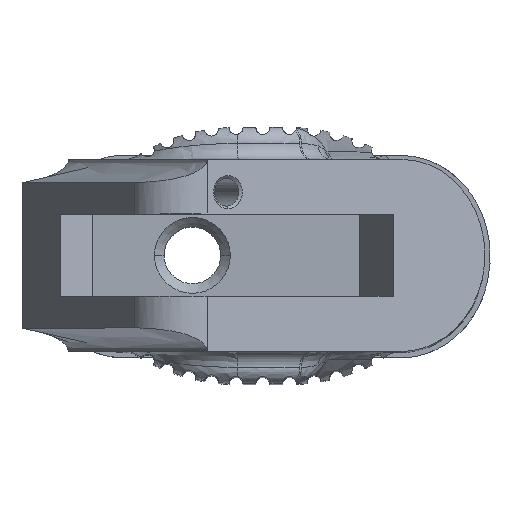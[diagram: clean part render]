
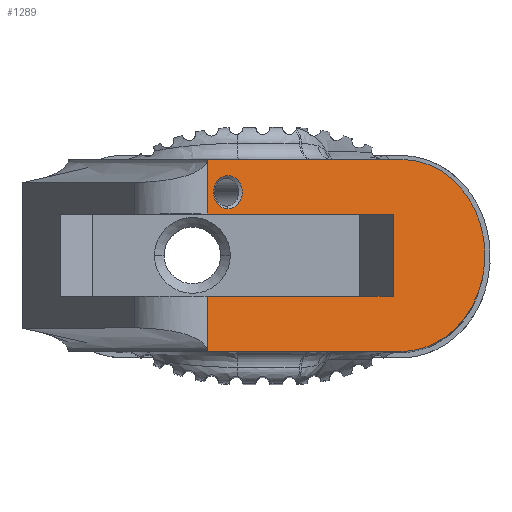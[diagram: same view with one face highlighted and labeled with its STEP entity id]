
A CAD part, top view. The second image highlights one B-rep face of the part: STEP entity #1289.
In plain terms, the highlighted planar face has unit normal (0.5, 0, 0.866).
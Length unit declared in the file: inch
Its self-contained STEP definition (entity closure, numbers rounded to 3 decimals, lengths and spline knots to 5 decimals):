
#49 = CARTESIAN_POINT ( 'NONE',  ( 0.64959, -1.00968, 2.3827 ) ) ;
#59 = CARTESIAN_POINT ( 'NONE',  ( 0.55214, -0.85579, 2.43896 ) ) ;
#67 = VERTEX_POINT ( 'NONE', #2289 ) ;
#109 = EDGE_CURVE ( 'NONE', #5710, #8721, #5941, .T. ) ;
#143 = CIRCLE ( 'NONE', #995, 0.07753 ) ;
#194 = LINE ( 'NONE', #4719, #1445 ) ;
#231 = VERTEX_POINT ( 'NONE', #6313 ) ;
#280 = CARTESIAN_POINT ( 'NONE',  ( 1.85118, -1.75318, 1.68896 ) ) ;
#450 = ORIENTED_EDGE ( 'NONE', *, *, #4851, .T. ) ;
#474 = CARTESIAN_POINT ( 'NONE',  ( 1.85118, -0.85518, 1.68896 ) ) ;
#483 = DIRECTION ( 'NONE',  ( 0., -1., 0. ) ) ;
#579 =( BOUNDED_CURVE ( )  B_SPLINE_CURVE ( 3, ( #3923, #6057, #5394, #5427 ),
 .UNSPECIFIED., .F., .F. ) 
 B_SPLINE_CURVE_WITH_KNOTS ( ( 4, 4 ),
 ( 0.00005, 0.01728 ),
 .UNSPECIFIED. ) 
 CURVE ( )  GEOMETRIC_REPRESENTATION_ITEM ( )  RATIONAL_B_SPLINE_CURVE ( ( 0.998, 0.813, 0.805, 0.974 ) ) 
 REPRESENTATION_ITEM ( '' )  );
#888 = VECTOR ( 'NONE', #2518, 39.37008 ) ;
#976 = ORIENTED_EDGE ( 'NONE', *, *, #3969, .T. ) ;
#995 = AXIS2_PLACEMENT_3D ( 'NONE', #3711, #8010, #5857 ) ;
#1004 = VECTOR ( 'NONE', #7785, 39.37008 ) ;
#1289 = ADVANCED_FACE ( 'NONE', ( #8086, #5645 ), #4890, .F. ) ;
#1362 = DIRECTION ( 'NONE',  ( -0.5, 0., -0.866 ) ) ;
#1391 = ORIENTED_EDGE ( 'NONE', *, *, #4881, .F. ) ;
#1445 = VECTOR ( 'NONE', #6880, 39.37008 ) ;
#1449 = CARTESIAN_POINT ( 'NONE',  ( 0.55214, -1.11168, 2.43896 ) ) ;
#1474 = ORIENTED_EDGE ( 'NONE', *, *, #6760, .F. ) ;
#1552 = ORIENTED_EDGE ( 'NONE', *, *, #109, .F. ) ;
#1583 = VERTEX_POINT ( 'NONE', #5786 ) ;
#1841 = CARTESIAN_POINT ( 'NONE',  ( 0.55214, -1.64468, 2.43896 ) ) ;
#1843 = CARTESIAN_POINT ( 'NONE',  ( 1.42249, -1.64468, 1.93646 ) ) ;
#1896 = DIRECTION ( 'NONE',  ( 0., 1., 0. ) ) ;
#1909 = EDGE_CURVE ( 'NONE', #1583, #3276, #7645, .T. ) ;
#1973 = ORIENTED_EDGE ( 'NONE', *, *, #1909, .F. ) ;
#2002 = VECTOR ( 'NONE', #4717, 39.37008 ) ;
#2034 = CARTESIAN_POINT ( 'NONE',  ( 1.46406, -1.75318, 1.91246 ) ) ;
#2087 = CARTESIAN_POINT ( 'NONE',  ( 0.64959, -0.93215, 2.3827 ) ) ;
#2289 = CARTESIAN_POINT ( 'NONE',  ( 0.55214, -1.75257, 2.43896 ) ) ;
#2511 = CARTESIAN_POINT ( 'NONE',  ( 0.55214, -1.11168, 2.43896 ) ) ;
#2518 = DIRECTION ( 'NONE',  ( 0., -1., 0. ) ) ;
#2566 = CARTESIAN_POINT ( 'NONE',  ( 1.83672, -1.58367, 1.69731 ) ) ;
#2588 = DIRECTION ( 'NONE',  ( -0.866, 0., 0.5 ) ) ;
#2613 = EDGE_CURVE ( 'NONE', #4546, #2988, #143, .T. ) ;
#2888 = DIRECTION ( 'NONE',  ( -0.5, 0., -0.866 ) ) ;
#2901 = VERTEX_POINT ( 'NONE', #7061 ) ;
#2966 = ORIENTED_EDGE ( 'NONE', *, *, #8639, .T. ) ;
#2988 = VERTEX_POINT ( 'NONE', #2087 ) ;
#3011 = ORIENTED_EDGE ( 'NONE', *, *, #2613, .T. ) ;
#3178 = DIRECTION ( 'NONE',  ( -0.866, 0., 0.5 ) ) ;
#3276 = VERTEX_POINT ( 'NONE', #5610 ) ;
#3422 = ORIENTED_EDGE ( 'NONE', *, *, #8412, .T. ) ;
#3426 = CARTESIAN_POINT ( 'NONE',  ( 1.67849, -1.75263, 1.78866 ) ) ;
#3581 = DIRECTION ( 'NONE',  ( 0., 1., 0. ) ) ;
#3589 = AXIS2_PLACEMENT_3D ( 'NONE', #49, #2888, #3581 ) ;
#3665 = VECTOR ( 'NONE', #1896, 39.37008 ) ;
#3711 = CARTESIAN_POINT ( 'NONE',  ( 0.64959, -1.00968, 2.3827 ) ) ;
#3923 = CARTESIAN_POINT ( 'NONE',  ( 1.46406, -0.85518, 1.91246 ) ) ;
#3969 = EDGE_CURVE ( 'NONE', #67, #8041, #8507, .T. ) ;
#4009 = LINE ( 'NONE', #4076, #3665 ) ;
#4034 = VECTOR ( 'NONE', #3178, 39.37008 ) ;
#4060 = CARTESIAN_POINT ( 'NONE',  ( 0.55214, -1.75318, 2.43896 ) ) ;
#4076 = CARTESIAN_POINT ( 'NONE',  ( 1.85118, -1.64468, 1.68896 ) ) ;
#4158 = CARTESIAN_POINT ( 'NONE',  ( 0.55214, -1.49668, 2.43896 ) ) ;
#4246 = LINE ( 'NONE', #5672, #6272 ) ;
#4460 = CIRCLE ( 'NONE', #3589, 0.07753 ) ;
#4546 = VERTEX_POINT ( 'NONE', #5006 ) ;
#4717 = DIRECTION ( 'NONE',  ( 0., -1., 0. ) ) ;
#4719 = CARTESIAN_POINT ( 'NONE',  ( 0.55214, -1.64468, 2.43896 ) ) ;
#4791 = LINE ( 'NONE', #474, #7398 ) ;
#4851 = EDGE_CURVE ( 'NONE', #8041, #3276, #5107, .T. ) ;
#4881 = EDGE_CURVE ( 'NONE', #67, #5576, #194, .T. ) ;
#4890 = PLANE ( 'NONE',  #7955 ) ;
#5006 = CARTESIAN_POINT ( 'NONE',  ( 0.64959, -1.08721, 2.3827 ) ) ;
#5018 = VECTOR ( 'NONE', #483, 39.37008 ) ;
#5107 = LINE ( 'NONE', #280, #7629 ) ;
#5146 = CARTESIAN_POINT ( 'NONE',  ( 1.42249, -1.11168, 1.93646 ) ) ;
#5150 = EDGE_LOOP ( 'NONE', ( #1973, #3422, #1474, #7064, #8268, #7145, #1552, #6837, #5519, #1391, #976, #450 ) ) ;
#5233 = VERTEX_POINT ( 'NONE', #59 ) ;
#5272 = VERTEX_POINT ( 'NONE', #6461 ) ;
#5274 = DIRECTION ( 'NONE',  ( 0.866, 0., -0.5 ) ) ;
#5394 = CARTESIAN_POINT ( 'NONE',  ( 1.83672, -1.02468, 1.69731 ) ) ;
#5427 = CARTESIAN_POINT ( 'NONE',  ( 1.85119, -1.27413, 1.68897 ) ) ;
#5519 = ORIENTED_EDGE ( 'NONE', *, *, #6070, .T. ) ;
#5576 = VERTEX_POINT ( 'NONE', #4158 ) ;
#5586 = LINE ( 'NONE', #1843, #5018 ) ;
#5610 = CARTESIAN_POINT ( 'NONE',  ( 1.46406, -1.75318, 1.91246 ) ) ;
#5627 = CARTESIAN_POINT ( 'NONE',  ( 0.55214, -1.49668, 2.43896 ) ) ;
#5645 = FACE_OUTER_BOUND ( 'NONE', #5150, .T. ) ;
#5672 = CARTESIAN_POINT ( 'NONE',  ( 0.55214, -1.64468, 2.43896 ) ) ;
#5710 = VERTEX_POINT ( 'NONE', #5146 ) ;
#5786 = CARTESIAN_POINT ( 'NONE',  ( 1.85119, -1.33423, 1.68897 ) ) ;
#5857 = DIRECTION ( 'NONE',  ( 0., 1., 0. ) ) ;
#5941 = LINE ( 'NONE', #2511, #4034 ) ;
#5971 = EDGE_CURVE ( 'NONE', #5272, #2901, #4791, .T. ) ;
#6023 = EDGE_CURVE ( 'NONE', #2901, #5233, #8719, .T. ) ;
#6057 = CARTESIAN_POINT ( 'NONE',  ( 1.67849, -0.85573, 1.78866 ) ) ;
#6070 = EDGE_CURVE ( 'NONE', #6770, #5576, #7950, .T. ) ;
#6085 = CARTESIAN_POINT ( 'NONE',  ( 0.55214, -0.96368, 2.43896 ) ) ;
#6157 = CARTESIAN_POINT ( 'NONE',  ( 1.42249, -1.49668, 1.93646 ) ) ;
#6172 = CARTESIAN_POINT ( 'NONE',  ( 1.85119, -1.33423, 1.68897 ) ) ;
#6272 = VECTOR ( 'NONE', #7756, 39.37008 ) ;
#6313 = CARTESIAN_POINT ( 'NONE',  ( 1.85119, -1.27413, 1.68897 ) ) ;
#6461 = CARTESIAN_POINT ( 'NONE',  ( 1.46406, -0.85518, 1.91246 ) ) ;
#6760 = EDGE_CURVE ( 'NONE', #5272, #231, #579, .T. ) ;
#6770 = VERTEX_POINT ( 'NONE', #6157 ) ;
#6837 = ORIENTED_EDGE ( 'NONE', *, *, #6990, .T. ) ;
#6880 = DIRECTION ( 'NONE',  ( 0., 1., 0. ) ) ;
#6990 = EDGE_CURVE ( 'NONE', #5710, #6770, #5586, .T. ) ;
#7061 = CARTESIAN_POINT ( 'NONE',  ( 0.55214, -0.85518, 2.43896 ) ) ;
#7064 = ORIENTED_EDGE ( 'NONE', *, *, #5971, .T. ) ;
#7120 = DIRECTION ( 'NONE',  ( 0., 1., 0. ) ) ;
#7145 = ORIENTED_EDGE ( 'NONE', *, *, #9166, .F. ) ;
#7398 = VECTOR ( 'NONE', #2588, 39.37008 ) ;
#7629 = VECTOR ( 'NONE', #5274, 39.37008 ) ;
#7645 =( BOUNDED_CURVE ( )  B_SPLINE_CURVE ( 3, ( #6172, #2566, #3426, #2034 ),
 .UNSPECIFIED., .F., .F. ) 
 B_SPLINE_CURVE_WITH_KNOTS ( ( 4, 4 ),
 ( 0., 0.01703 ),
 .UNSPECIFIED. ) 
 CURVE ( )  GEOMETRIC_REPRESENTATION_ITEM ( )  RATIONAL_B_SPLINE_CURVE ( ( 0.974, 0.805, 0.813, 0.998 ) ) 
 REPRESENTATION_ITEM ( '' )  );
#7756 = DIRECTION ( 'NONE',  ( 0., 1., 0. ) ) ;
#7785 = DIRECTION ( 'NONE',  ( -0.866, 0., 0.5 ) ) ;
#7950 = LINE ( 'NONE', #5627, #1004 ) ;
#7955 = AXIS2_PLACEMENT_3D ( 'NONE', #8459, #1362, #7120 ) ;
#8010 = DIRECTION ( 'NONE',  ( -0.5, 0., -0.866 ) ) ;
#8041 = VERTEX_POINT ( 'NONE', #4060 ) ;
#8086 = FACE_BOUND ( 'NONE', #8244, .T. ) ;
#8244 = EDGE_LOOP ( 'NONE', ( #3011, #2966 ) ) ;
#8268 = ORIENTED_EDGE ( 'NONE', *, *, #6023, .T. ) ;
#8412 = EDGE_CURVE ( 'NONE', #1583, #231, #4009, .T. ) ;
#8459 = CARTESIAN_POINT ( 'NONE',  ( 0.55214, -1.64468, 2.43896 ) ) ;
#8507 = LINE ( 'NONE', #1841, #2002 ) ;
#8639 = EDGE_CURVE ( 'NONE', #2988, #4546, #4460, .T. ) ;
#8719 = LINE ( 'NONE', #6085, #888 ) ;
#8721 = VERTEX_POINT ( 'NONE', #1449 ) ;
#9166 = EDGE_CURVE ( 'NONE', #8721, #5233, #4246, .T. ) ;
